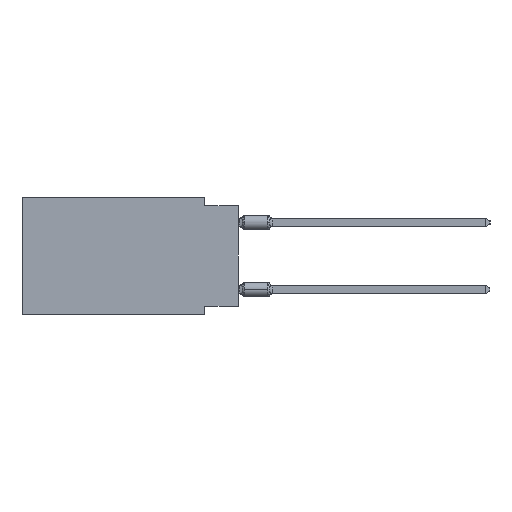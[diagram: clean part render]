
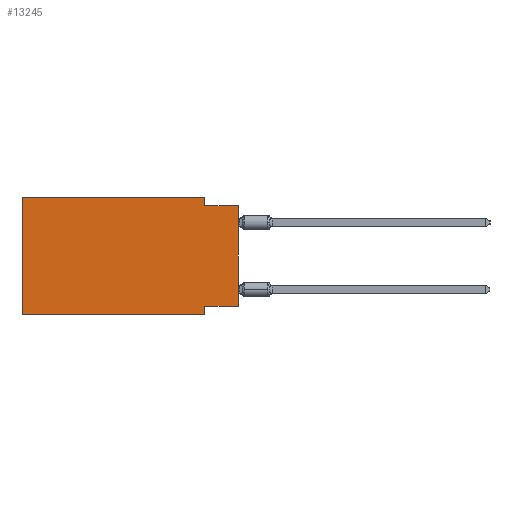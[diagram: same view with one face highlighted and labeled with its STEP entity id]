
A CAD part, left-side view. The second image highlights one B-rep face of the part: STEP entity #13245.
In plain terms, the highlighted planar face has unit normal (-1, 0, 0).
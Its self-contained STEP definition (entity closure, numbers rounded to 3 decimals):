
#25 = EDGE_CURVE ( 'NONE', #53706, #34473, #29845, .T. ) ;
#3176 = CARTESIAN_POINT ( 'NONE',  ( 0., 0., -0.635 ) ) ;
#4489 = VERTEX_POINT ( 'NONE', #18887 ) ;
#5004 = EDGE_CURVE ( 'NONE', #4489, #39852, #10826, .T. ) ;
#9017 = CARTESIAN_POINT ( 'NONE',  ( 0., 0., -8.255 ) ) ;
#9099 = DIRECTION ( 'NONE',  ( 0., -1., 0. ) ) ;
#9819 = CARTESIAN_POINT ( 'NONE',  ( 0., 2.54, 0. ) ) ;
#10658 = DIRECTION ( 'NONE',  ( 1., 0., 0. ) ) ;
#10757 = LINE ( 'NONE', #59166, #40700 ) ;
#10826 = LINE ( 'NONE', #16376, #57231 ) ;
#11329 = DIRECTION ( 'NONE',  ( 0., -1., 0. ) ) ;
#13245 = ADVANCED_FACE ( 'NONE', ( #52321 ), #30110, .F. ) ;
#13937 = LINE ( 'NONE', #28156, #55407 ) ;
#15727 = VERTEX_POINT ( 'NONE', #9819 ) ;
#16376 = CARTESIAN_POINT ( 'NONE',  ( 0., 0., -0.635 ) ) ;
#16471 = LINE ( 'NONE', #50074, #50706 ) ;
#17030 = CARTESIAN_POINT ( 'NONE',  ( 0., 0., 0. ) ) ;
#18622 = CARTESIAN_POINT ( 'NONE',  ( 0., 16.383, -8.89 ) ) ;
#18887 = CARTESIAN_POINT ( 'NONE',  ( 0., 2.54, -0.635 ) ) ;
#20742 = LINE ( 'NONE', #17030, #40587 ) ;
#22554 = EDGE_CURVE ( 'NONE', #15727, #4489, #54074, .T. ) ;
#25669 = DIRECTION ( 'NONE',  ( 0., 0., 1. ) ) ;
#27515 = DIRECTION ( 'NONE',  ( 0., 1., 0. ) ) ;
#28017 = EDGE_CURVE ( 'NONE', #31421, #39852, #20742, .T. ) ;
#28156 = CARTESIAN_POINT ( 'NONE',  ( 0., 0., -8.255 ) ) ;
#29845 = LINE ( 'NONE', #53610, #35700 ) ;
#29897 = CARTESIAN_POINT ( 'NONE',  ( 0., 16.383, 0. ) ) ;
#30048 = DIRECTION ( 'NONE',  ( 0., 0., -1. ) ) ;
#30110 = PLANE ( 'NONE',  #59159 ) ;
#30975 = DIRECTION ( 'NONE',  ( 0., 0., -1. ) ) ;
#31421 = VERTEX_POINT ( 'NONE', #9017 ) ;
#31643 = CARTESIAN_POINT ( 'NONE',  ( 0., 16.383, 0. ) ) ;
#34473 = VERTEX_POINT ( 'NONE', #55292 ) ;
#35700 = VECTOR ( 'NONE', #11329, 1000. ) ;
#35734 = DIRECTION ( 'NONE',  ( 0., 0., 1. ) ) ;
#37053 = CARTESIAN_POINT ( 'NONE',  ( 0., 2.54, -8.255 ) ) ;
#38314 = EDGE_CURVE ( 'NONE', #31421, #48269, #13937, .T. ) ;
#38423 = CARTESIAN_POINT ( 'NONE',  ( 0., 16.383, 0. ) ) ;
#38500 = ORIENTED_EDGE ( 'NONE', *, *, #5004, .F. ) ;
#39030 = EDGE_CURVE ( 'NONE', #53706, #51782, #10757, .T. ) ;
#39248 = ORIENTED_EDGE ( 'NONE', *, *, #38314, .F. ) ;
#39852 = VERTEX_POINT ( 'NONE', #3176 ) ;
#39907 = CARTESIAN_POINT ( 'NONE',  ( 0., 2.54, 0. ) ) ;
#40587 = VECTOR ( 'NONE', #25669, 1000. ) ;
#40700 = VECTOR ( 'NONE', #35734, 1000. ) ;
#42283 = ORIENTED_EDGE ( 'NONE', *, *, #28017, .T. ) ;
#43206 = EDGE_LOOP ( 'NONE', ( #42283, #38500, #59716, #59082, #61009, #60981, #56863, #39248 ) ) ;
#44446 = DIRECTION ( 'NONE',  ( 0., -1., 0. ) ) ;
#48017 = DIRECTION ( 'NONE',  ( 0., 0., -1. ) ) ;
#48269 = VERTEX_POINT ( 'NONE', #37053 ) ;
#49006 = EDGE_CURVE ( 'NONE', #51782, #15727, #60337, .T. ) ;
#50074 = CARTESIAN_POINT ( 'NONE',  ( 0., 2.54, -8.89 ) ) ;
#50706 = VECTOR ( 'NONE', #30975, 1000. ) ;
#51782 = VERTEX_POINT ( 'NONE', #29897 ) ;
#52321 = FACE_OUTER_BOUND ( 'NONE', #43206, .T. ) ;
#53610 = CARTESIAN_POINT ( 'NONE',  ( 0., 16.383, -8.89 ) ) ;
#53706 = VERTEX_POINT ( 'NONE', #18622 ) ;
#54074 = LINE ( 'NONE', #39907, #58380 ) ;
#55292 = CARTESIAN_POINT ( 'NONE',  ( 0., 2.54, -8.89 ) ) ;
#55407 = VECTOR ( 'NONE', #27515, 1000. ) ;
#56265 = EDGE_CURVE ( 'NONE', #48269, #34473, #16471, .T. ) ;
#56863 = ORIENTED_EDGE ( 'NONE', *, *, #56265, .F. ) ;
#57231 = VECTOR ( 'NONE', #44446, 1000. ) ;
#58380 = VECTOR ( 'NONE', #30048, 1000. ) ;
#58464 = VECTOR ( 'NONE', #9099, 1000. ) ;
#59082 = ORIENTED_EDGE ( 'NONE', *, *, #49006, .F. ) ;
#59159 = AXIS2_PLACEMENT_3D ( 'NONE', #38423, #10658, #48017 ) ;
#59166 = CARTESIAN_POINT ( 'NONE',  ( 0., 16.383, 0. ) ) ;
#59716 = ORIENTED_EDGE ( 'NONE', *, *, #22554, .F. ) ;
#60337 = LINE ( 'NONE', #31643, #58464 ) ;
#60981 = ORIENTED_EDGE ( 'NONE', *, *, #25, .T. ) ;
#61009 = ORIENTED_EDGE ( 'NONE', *, *, #39030, .F. ) ;
